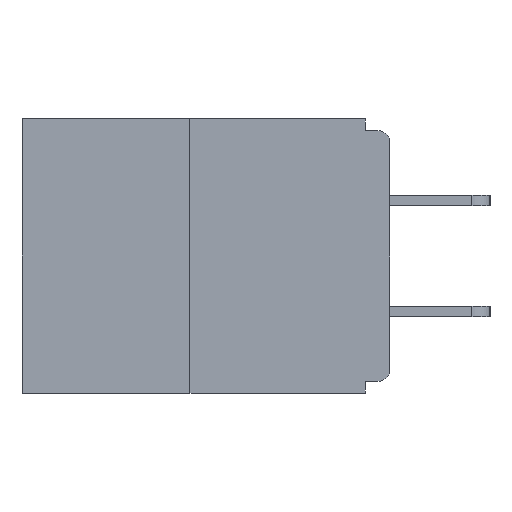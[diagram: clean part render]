
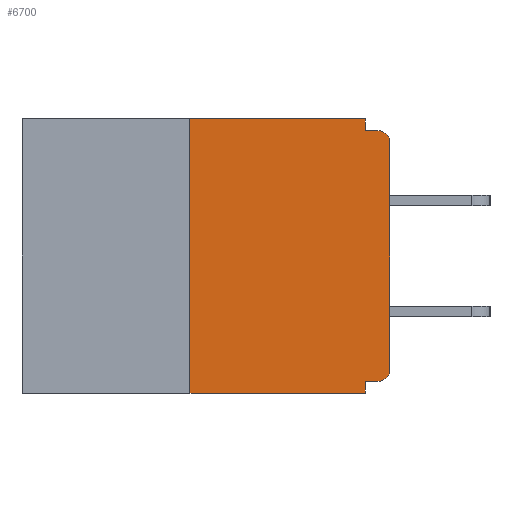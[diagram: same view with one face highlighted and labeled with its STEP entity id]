
A CAD part, left-side view. The second image highlights one B-rep face of the part: STEP entity #6700.
In plain terms, the highlighted planar face has unit normal (-1, 0, 0).
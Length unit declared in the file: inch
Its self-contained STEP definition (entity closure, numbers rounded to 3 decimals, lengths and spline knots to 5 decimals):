
#12 = LINE ( 'NONE', #2844, #984 ) ;
#156 = EDGE_CURVE ( 'NONE', #12075, #4788, #8591, .T. ) ;
#349 = ORIENTED_EDGE ( 'NONE', *, *, #7680, .F. ) ;
#445 = DIRECTION ( 'NONE',  ( 0., 0., -1. ) ) ;
#586 = AXIS2_PLACEMENT_3D ( 'NONE', #11264, #1085, #6497 ) ;
#599 = LINE ( 'NONE', #3396, #10975 ) ;
#711 = DIRECTION ( 'NONE',  ( 0., 0., 1. ) ) ;
#820 = CARTESIAN_POINT ( 'NONE',  ( 0., 0.031, -0.015 ) ) ;
#984 = VECTOR ( 'NONE', #2785, 39.37008 ) ;
#1004 = CARTESIAN_POINT ( 'NONE',  ( 0., 0.015, -0.015 ) ) ;
#1055 = DIRECTION ( 'NONE',  ( 0., 0., -1. ) ) ;
#1085 = DIRECTION ( 'NONE',  ( -1., 0., 0. ) ) ;
#1207 = DIRECTION ( 'NONE',  ( 0., -1., 0. ) ) ;
#1389 = CARTESIAN_POINT ( 'NONE',  ( 0., 0.46, 0. ) ) ;
#1673 = VECTOR ( 'NONE', #7148, 39.37008 ) ;
#1675 = VERTEX_POINT ( 'NONE', #10007 ) ;
#2028 = DIRECTION ( 'NONE',  ( 0., 0., -1. ) ) ;
#2139 = ORIENTED_EDGE ( 'NONE', *, *, #6434, .F. ) ;
#2306 = CARTESIAN_POINT ( 'NONE',  ( 0., 0.015, -0.328 ) ) ;
#2315 = VERTEX_POINT ( 'NONE', #9558 ) ;
#2468 = DIRECTION ( 'NONE',  ( 0., 0., -1. ) ) ;
#2611 = EDGE_CURVE ( 'NONE', #4197, #11646, #10850, .T. ) ;
#2785 = DIRECTION ( 'NONE',  ( 0., -1., 0. ) ) ;
#2844 = CARTESIAN_POINT ( 'NONE',  ( 0., 0., -0.015 ) ) ;
#3101 = ORIENTED_EDGE ( 'NONE', *, *, #2611, .F. ) ;
#3355 = LINE ( 'NONE', #1389, #1673 ) ;
#3396 = CARTESIAN_POINT ( 'NONE',  ( 0., 0., 0. ) ) ;
#3689 = VECTOR ( 'NONE', #2468, 39.37008 ) ;
#3730 = EDGE_CURVE ( 'NONE', #11646, #7746, #12, .T. ) ;
#3822 = CARTESIAN_POINT ( 'NONE',  ( 0., 0.031, -0.343 ) ) ;
#4017 = ORIENTED_EDGE ( 'NONE', *, *, #156, .T. ) ;
#4197 = VERTEX_POINT ( 'NONE', #4805 ) ;
#4241 = EDGE_CURVE ( 'NONE', #4487, #7746, #6545, .T. ) ;
#4485 = EDGE_CURVE ( 'NONE', #2315, #4197, #3355, .T. ) ;
#4487 = VERTEX_POINT ( 'NONE', #5260 ) ;
#4703 = AXIS2_PLACEMENT_3D ( 'NONE', #5107, #11640, #445 ) ;
#4788 = VERTEX_POINT ( 'NONE', #6943 ) ;
#4805 = CARTESIAN_POINT ( 'NONE',  ( 0., 0.031, 0. ) ) ;
#5086 = VERTEX_POINT ( 'NONE', #9009 ) ;
#5107 = CARTESIAN_POINT ( 'NONE',  ( 0., 0.46, 0. ) ) ;
#5260 = CARTESIAN_POINT ( 'NONE',  ( 0., 0., -0.03 ) ) ;
#5542 = ORIENTED_EDGE ( 'NONE', *, *, #10466, .T. ) ;
#5581 = VECTOR ( 'NONE', #1207, 39.37008 ) ;
#5819 = EDGE_CURVE ( 'NONE', #1675, #5086, #10244, .T. ) ;
#5924 = LINE ( 'NONE', #10578, #5581 ) ;
#6015 = DIRECTION ( 'NONE',  ( 0., 0., 1. ) ) ;
#6196 = VECTOR ( 'NONE', #711, 39.37008 ) ;
#6434 = EDGE_CURVE ( 'NONE', #9997, #2315, #9126, .T. ) ;
#6470 = CARTESIAN_POINT ( 'NONE',  ( 0., 0., -0.328 ) ) ;
#6497 = DIRECTION ( 'NONE',  ( 0., 0., -1. ) ) ;
#6510 = CARTESIAN_POINT ( 'NONE',  ( 0., 0.25, -0.343 ) ) ;
#6545 = CIRCLE ( 'NONE', #11904, 0.015 ) ;
#6700 = ADVANCED_FACE ( 'NONE', ( #9845 ), #11831, .F. ) ;
#6781 = ORIENTED_EDGE ( 'NONE', *, *, #4241, .T. ) ;
#6943 = CARTESIAN_POINT ( 'NONE',  ( 0., 0., -0.313 ) ) ;
#7148 = DIRECTION ( 'NONE',  ( 0., -1., 0. ) ) ;
#7505 = EDGE_LOOP ( 'NONE', ( #9959, #2139, #5542, #11839, #349, #4017, #11612, #6781, #10000, #3101 ) ) ;
#7680 = EDGE_CURVE ( 'NONE', #12075, #1675, #11045, .T. ) ;
#7746 = VERTEX_POINT ( 'NONE', #1004 ) ;
#8238 = CARTESIAN_POINT ( 'NONE',  ( 0., 0.25, 0. ) ) ;
#8356 = DIRECTION ( 'NONE',  ( -1., 0., 0. ) ) ;
#8588 = VECTOR ( 'NONE', #12099, 39.37008 ) ;
#8591 = CIRCLE ( 'NONE', #586, 0.015 ) ;
#8981 = VECTOR ( 'NONE', #1055, 39.37008 ) ;
#8992 = CARTESIAN_POINT ( 'NONE',  ( 0., 0.031, 0. ) ) ;
#9009 = CARTESIAN_POINT ( 'NONE',  ( 0., 0.031, -0.343 ) ) ;
#9126 = LINE ( 'NONE', #8238, #6196 ) ;
#9558 = CARTESIAN_POINT ( 'NONE',  ( 0., 0.25, 0. ) ) ;
#9845 = FACE_OUTER_BOUND ( 'NONE', #7505, .T. ) ;
#9959 = ORIENTED_EDGE ( 'NONE', *, *, #4485, .F. ) ;
#9997 = VERTEX_POINT ( 'NONE', #6510 ) ;
#10000 = ORIENTED_EDGE ( 'NONE', *, *, #3730, .F. ) ;
#10007 = CARTESIAN_POINT ( 'NONE',  ( 0., 0.031, -0.328 ) ) ;
#10244 = LINE ( 'NONE', #3822, #8981 ) ;
#10466 = EDGE_CURVE ( 'NONE', #9997, #5086, #5924, .T. ) ;
#10578 = CARTESIAN_POINT ( 'NONE',  ( 0., 0.46, -0.343 ) ) ;
#10850 = LINE ( 'NONE', #8992, #3689 ) ;
#10975 = VECTOR ( 'NONE', #6015, 39.37008 ) ;
#11045 = LINE ( 'NONE', #6470, #8588 ) ;
#11264 = CARTESIAN_POINT ( 'NONE',  ( 0., 0.015, -0.313 ) ) ;
#11431 = EDGE_CURVE ( 'NONE', #4788, #4487, #599, .T. ) ;
#11457 = CARTESIAN_POINT ( 'NONE',  ( 0., 0.015, -0.03 ) ) ;
#11612 = ORIENTED_EDGE ( 'NONE', *, *, #11431, .T. ) ;
#11640 = DIRECTION ( 'NONE',  ( 1., 0., 0. ) ) ;
#11646 = VERTEX_POINT ( 'NONE', #820 ) ;
#11831 = PLANE ( 'NONE',  #4703 ) ;
#11839 = ORIENTED_EDGE ( 'NONE', *, *, #5819, .F. ) ;
#11904 = AXIS2_PLACEMENT_3D ( 'NONE', #11457, #8356, #2028 ) ;
#12075 = VERTEX_POINT ( 'NONE', #2306 ) ;
#12099 = DIRECTION ( 'NONE',  ( 0., 1., 0. ) ) ;
